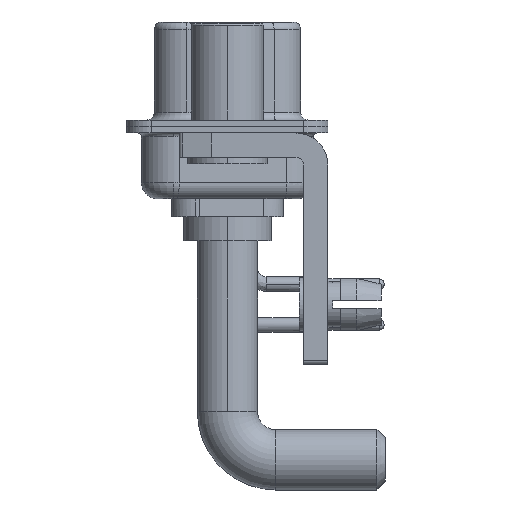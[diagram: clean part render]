
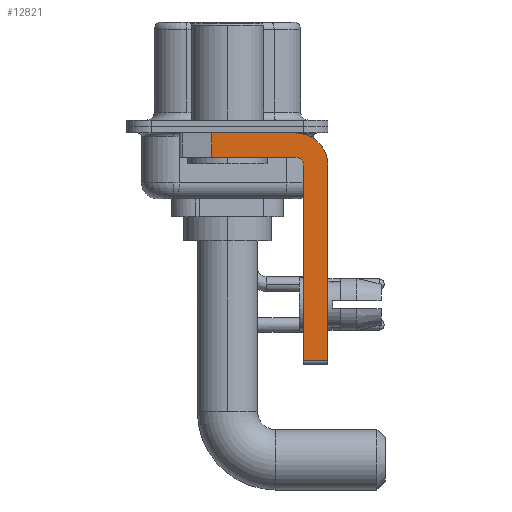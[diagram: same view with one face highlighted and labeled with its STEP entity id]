
A CAD part, left-side view. The second image highlights one B-rep face of the part: STEP entity #12821.
In plain terms, the highlighted planar face has unit normal (-1, 0, 0).
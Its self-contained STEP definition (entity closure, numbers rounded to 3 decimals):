
#751 = VERTEX_POINT ( 'NONE', #13732 ) ;
#835 = CIRCLE ( 'NONE', #1295, 2. ) ;
#1167 = FACE_OUTER_BOUND ( 'NONE', #4259, .T. ) ;
#1295 = AXIS2_PLACEMENT_3D ( 'NONE', #2947, #6922, #11940 ) ;
#1610 = ORIENTED_EDGE ( 'NONE', *, *, #6810, .F. ) ;
#1924 = CARTESIAN_POINT ( 'NONE',  ( -2.9, 0.978, -0.4 ) ) ;
#1951 = LINE ( 'NONE', #13013, #11480 ) ;
#2300 = CARTESIAN_POINT ( 'NONE',  ( -2.9, -4.25, -0.4 ) ) ;
#2405 = VERTEX_POINT ( 'NONE', #22142 ) ;
#2947 = CARTESIAN_POINT ( 'NONE',  ( -2.9, -4.25, -2.4 ) ) ;
#3967 = LINE ( 'NONE', #19893, #24850 ) ;
#4259 = EDGE_LOOP ( 'NONE', ( #18001, #8556, #8264, #1610, #16691, #20642, #28303, #12676 ) ) ;
#4349 = CARTESIAN_POINT ( 'NONE',  ( -2.9, 3., -0.4 ) ) ;
#4644 = DIRECTION ( 'NONE',  ( 0., -1., 0. ) ) ;
#4823 = CARTESIAN_POINT ( 'NONE',  ( -2.9, 0.978, -1.9 ) ) ;
#4879 = VERTEX_POINT ( 'NONE', #16890 ) ;
#5099 = EDGE_CURVE ( 'NONE', #21367, #11774, #16122, .T. ) ;
#6256 = AXIS2_PLACEMENT_3D ( 'NONE', #12440, #10220, #19234 ) ;
#6459 = CARTESIAN_POINT ( 'NONE',  ( -2.9, -4.25, -1.9 ) ) ;
#6810 = EDGE_CURVE ( 'NONE', #751, #21367, #19937, .T. ) ;
#6922 = DIRECTION ( 'NONE',  ( 1., 0., 0. ) ) ;
#7913 = VECTOR ( 'NONE', #9504, 1000. ) ;
#8264 = ORIENTED_EDGE ( 'NONE', *, *, #5099, .F. ) ;
#8556 = ORIENTED_EDGE ( 'NONE', *, *, #9299, .T. ) ;
#8820 = DIRECTION ( 'NONE',  ( 0., 0., -1. ) ) ;
#9299 = EDGE_CURVE ( 'NONE', #29183, #11774, #13245, .T. ) ;
#9504 = DIRECTION ( 'NONE',  ( 0., 1., 0. ) ) ;
#10152 = PLANE ( 'NONE',  #15890 ) ;
#10220 = DIRECTION ( 'NONE',  ( -1., 0., 0. ) ) ;
#10557 = EDGE_CURVE ( 'NONE', #4879, #2405, #3967, .T. ) ;
#11170 = DIRECTION ( 'NONE',  ( 1., 0., 0. ) ) ;
#11480 = VECTOR ( 'NONE', #22313, 1000. ) ;
#11774 = VERTEX_POINT ( 'NONE', #4823 ) ;
#11940 = DIRECTION ( 'NONE',  ( 0., 0., -1. ) ) ;
#12440 = CARTESIAN_POINT ( 'NONE',  ( -2.9, -4.25, -2.4 ) ) ;
#12668 = EDGE_CURVE ( 'NONE', #25436, #14760, #835, .T. ) ;
#12676 = ORIENTED_EDGE ( 'NONE', *, *, #12668, .F. ) ;
#12821 = ADVANCED_FACE ( 'NONE', ( #1167 ), #10152, .F. ) ;
#13008 = VECTOR ( 'NONE', #8820, 1000. ) ;
#13013 = CARTESIAN_POINT ( 'NONE',  ( -2.9, -6.25, -2.4 ) ) ;
#13245 = LINE ( 'NONE', #20486, #13008 ) ;
#13732 = CARTESIAN_POINT ( 'NONE',  ( -2.9, -4.75, -2.4 ) ) ;
#14462 = CARTESIAN_POINT ( 'NONE',  ( -2.9, -4.75, -14.8 ) ) ;
#14748 = LINE ( 'NONE', #14462, #28550 ) ;
#14760 = VERTEX_POINT ( 'NONE', #20449 ) ;
#15890 = AXIS2_PLACEMENT_3D ( 'NONE', #19162, #11170, #22405 ) ;
#16122 = LINE ( 'NONE', #24886, #7913 ) ;
#16691 = ORIENTED_EDGE ( 'NONE', *, *, #28955, .F. ) ;
#16890 = CARTESIAN_POINT ( 'NONE',  ( -2.9, -4.75, -14.55 ) ) ;
#17084 = DIRECTION ( 'NONE',  ( 0., -1., 0. ) ) ;
#18001 = ORIENTED_EDGE ( 'NONE', *, *, #28103, .F. ) ;
#19162 = CARTESIAN_POINT ( 'NONE',  ( -2.9, -4.25, -2.4 ) ) ;
#19234 = DIRECTION ( 'NONE',  ( 0., 0., 1. ) ) ;
#19893 = CARTESIAN_POINT ( 'NONE',  ( -2.9, -4.25, -14.55 ) ) ;
#19937 = CIRCLE ( 'NONE', #6256, 0.5 ) ;
#20449 = CARTESIAN_POINT ( 'NONE',  ( -2.9, -6.25, -2.4 ) ) ;
#20486 = CARTESIAN_POINT ( 'NONE',  ( -2.9, 0.978, -1.9 ) ) ;
#20642 = ORIENTED_EDGE ( 'NONE', *, *, #10557, .T. ) ;
#21367 = VERTEX_POINT ( 'NONE', #6459 ) ;
#21707 = DIRECTION ( 'NONE',  ( 0., 0., 1. ) ) ;
#22142 = CARTESIAN_POINT ( 'NONE',  ( -2.9, -6.25, -14.55 ) ) ;
#22313 = DIRECTION ( 'NONE',  ( 0., 0., -1. ) ) ;
#22405 = DIRECTION ( 'NONE',  ( 0., 0., -1. ) ) ;
#23570 = LINE ( 'NONE', #4349, #28512 ) ;
#24850 = VECTOR ( 'NONE', #17084, 1000. ) ;
#24886 = CARTESIAN_POINT ( 'NONE',  ( -2.9, -4.25, -1.9 ) ) ;
#25436 = VERTEX_POINT ( 'NONE', #2300 ) ;
#27233 = EDGE_CURVE ( 'NONE', #14760, #2405, #1951, .T. ) ;
#28103 = EDGE_CURVE ( 'NONE', #29183, #25436, #23570, .T. ) ;
#28303 = ORIENTED_EDGE ( 'NONE', *, *, #27233, .F. ) ;
#28512 = VECTOR ( 'NONE', #4644, 1000. ) ;
#28550 = VECTOR ( 'NONE', #21707, 1000. ) ;
#28955 = EDGE_CURVE ( 'NONE', #4879, #751, #14748, .T. ) ;
#29183 = VERTEX_POINT ( 'NONE', #1924 ) ;
